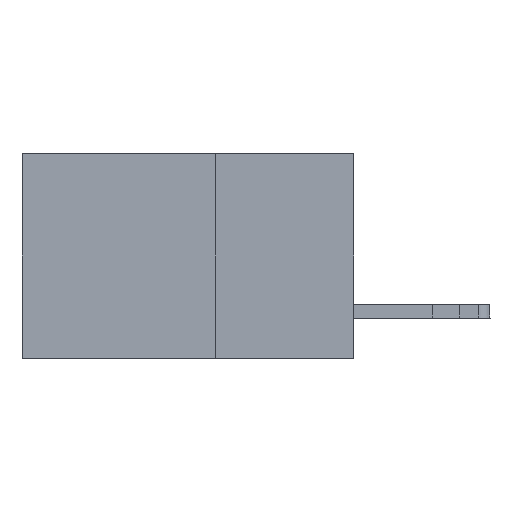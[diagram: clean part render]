
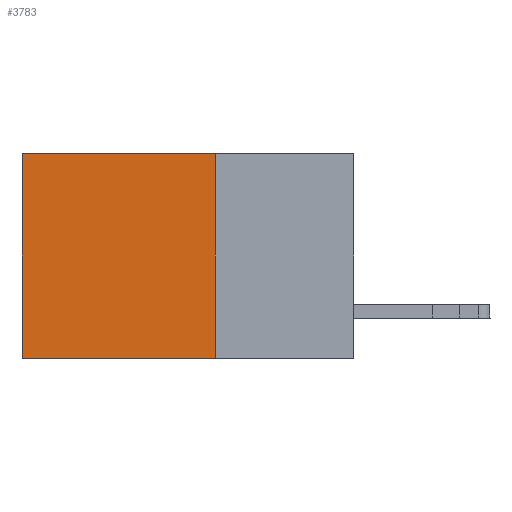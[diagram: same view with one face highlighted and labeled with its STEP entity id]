
A CAD part, left-side view. The second image highlights one B-rep face of the part: STEP entity #3783.
In plain terms, the highlighted planar face has unit normal (-1, 0, 0).
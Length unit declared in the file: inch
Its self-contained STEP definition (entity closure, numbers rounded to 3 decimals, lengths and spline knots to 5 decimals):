
#206 = ORIENTED_EDGE ( 'NONE', *, *, #14067, .F. ) ;
#3130 = CARTESIAN_POINT ( 'NONE',  ( 0.2875, 0.25, -0.37 ) ) ;
#3783 = ADVANCED_FACE ( 'NONE', ( #11721 ), #23425, .F. ) ;
#3971 = LINE ( 'NONE', #16433, #17848 ) ;
#4089 = CARTESIAN_POINT ( 'NONE',  ( 0.2875, 0.6, -0.37 ) ) ;
#5811 = LINE ( 'NONE', #7130, #19686 ) ;
#6064 = DIRECTION ( 'NONE',  ( 0., 1., 0. ) ) ;
#7130 = CARTESIAN_POINT ( 'NONE',  ( 0.2875, 0.6, 0. ) ) ;
#7659 = DIRECTION ( 'NONE',  ( 0., 0., -1. ) ) ;
#7930 = EDGE_CURVE ( 'NONE', #8542, #14266, #11523, .T. ) ;
#8479 = AXIS2_PLACEMENT_3D ( 'NONE', #16303, #18270, #21523 ) ;
#8542 = VERTEX_POINT ( 'NONE', #15577 ) ;
#8613 = VERTEX_POINT ( 'NONE', #4089 ) ;
#9993 = EDGE_LOOP ( 'NONE', ( #11812, #206, #12367, #17788 ) ) ;
#10837 = DIRECTION ( 'NONE',  ( 0., 0., -1. ) ) ;
#11523 = LINE ( 'NONE', #14863, #21448 ) ;
#11721 = FACE_OUTER_BOUND ( 'NONE', #9993, .T. ) ;
#11812 = ORIENTED_EDGE ( 'NONE', *, *, #11846, .T. ) ;
#11846 = EDGE_CURVE ( 'NONE', #16403, #8613, #5811, .T. ) ;
#12367 = ORIENTED_EDGE ( 'NONE', *, *, #7930, .F. ) ;
#14067 = EDGE_CURVE ( 'NONE', #14266, #8613, #3971, .T. ) ;
#14266 = VERTEX_POINT ( 'NONE', #3130 ) ;
#14501 = LINE ( 'NONE', #16737, #15349 ) ;
#14849 = DIRECTION ( 'NONE',  ( 0., 1., 0. ) ) ;
#14863 = CARTESIAN_POINT ( 'NONE',  ( 0.2875, 0.25, 0. ) ) ;
#15349 = VECTOR ( 'NONE', #6064, 39.37008 ) ;
#15577 = CARTESIAN_POINT ( 'NONE',  ( 0.2875, 0.25, 0. ) ) ;
#16126 = CARTESIAN_POINT ( 'NONE',  ( 0.2875, 0.6, 0. ) ) ;
#16303 = CARTESIAN_POINT ( 'NONE',  ( 0.2875, 0.25, 0. ) ) ;
#16403 = VERTEX_POINT ( 'NONE', #16126 ) ;
#16433 = CARTESIAN_POINT ( 'NONE',  ( 0.2875, 0.25, -0.37 ) ) ;
#16737 = CARTESIAN_POINT ( 'NONE',  ( 0.2875, 0.25, 0. ) ) ;
#17162 = EDGE_CURVE ( 'NONE', #8542, #16403, #14501, .T. ) ;
#17788 = ORIENTED_EDGE ( 'NONE', *, *, #17162, .T. ) ;
#17848 = VECTOR ( 'NONE', #14849, 39.37008 ) ;
#18270 = DIRECTION ( 'NONE',  ( 1., 0., 0. ) ) ;
#19686 = VECTOR ( 'NONE', #10837, 39.37008 ) ;
#21448 = VECTOR ( 'NONE', #7659, 39.37008 ) ;
#21523 = DIRECTION ( 'NONE',  ( 0., 0., -1. ) ) ;
#23425 = PLANE ( 'NONE',  #8479 ) ;
